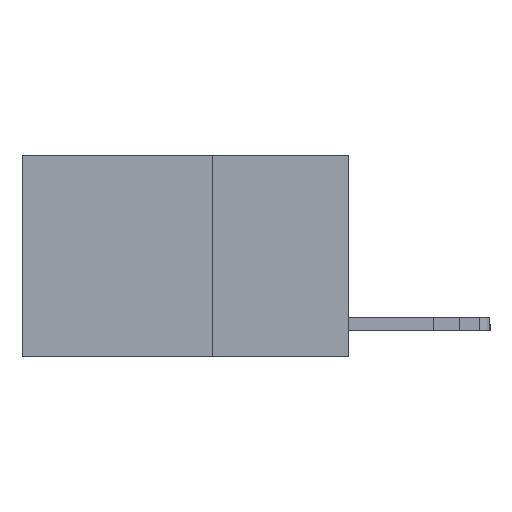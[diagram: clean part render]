
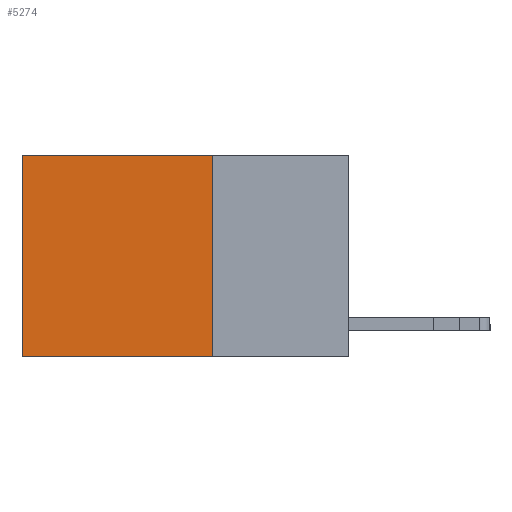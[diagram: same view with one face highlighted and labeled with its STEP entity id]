
A CAD part, left-side view. The second image highlights one B-rep face of the part: STEP entity #5274.
In plain terms, the highlighted planar face has unit normal (-1, 0, 0).
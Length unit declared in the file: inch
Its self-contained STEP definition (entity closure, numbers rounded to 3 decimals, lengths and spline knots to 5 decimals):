
#613 = VERTEX_POINT ( 'NONE', #13462 ) ;
#965 = CARTESIAN_POINT ( 'NONE',  ( 0.2625, 0.25, 0. ) ) ;
#1914 = EDGE_CURVE ( 'NONE', #18577, #613, #13755, .T. ) ;
#2426 = AXIS2_PLACEMENT_3D ( 'NONE', #17594, #7298, #4299 ) ;
#2745 = VECTOR ( 'NONE', #12208, 39.37008 ) ;
#2809 = LINE ( 'NONE', #18819, #14196 ) ;
#4299 = DIRECTION ( 'NONE',  ( 0., 0., -1. ) ) ;
#4348 = CARTESIAN_POINT ( 'NONE',  ( 0.2625, 0.25, -0.37 ) ) ;
#4615 = EDGE_CURVE ( 'NONE', #16564, #18577, #9957, .T. ) ;
#5274 = ADVANCED_FACE ( 'NONE', ( #11670 ), #14673, .F. ) ;
#5416 = DIRECTION ( 'NONE',  ( 0., 1., 0. ) ) ;
#7030 = EDGE_LOOP ( 'NONE', ( #14789, #12630, #12229, #9742 ) ) ;
#7270 = VECTOR ( 'NONE', #17537, 39.37008 ) ;
#7298 = DIRECTION ( 'NONE',  ( 1., 0., 0. ) ) ;
#7419 = EDGE_CURVE ( 'NONE', #11851, #613, #2809, .T. ) ;
#7636 = CARTESIAN_POINT ( 'NONE',  ( 0.2625, 0.6, 0. ) ) ;
#8005 = LINE ( 'NONE', #15856, #15349 ) ;
#9742 = ORIENTED_EDGE ( 'NONE', *, *, #4615, .T. ) ;
#9957 = LINE ( 'NONE', #18812, #7270 ) ;
#11670 = FACE_OUTER_BOUND ( 'NONE', #7030, .T. ) ;
#11851 = VERTEX_POINT ( 'NONE', #4348 ) ;
#12208 = DIRECTION ( 'NONE',  ( 0., 0., -1. ) ) ;
#12229 = ORIENTED_EDGE ( 'NONE', *, *, #16948, .F. ) ;
#12630 = ORIENTED_EDGE ( 'NONE', *, *, #7419, .F. ) ;
#13462 = CARTESIAN_POINT ( 'NONE',  ( 0.2625, 0.6, -0.37 ) ) ;
#13755 = LINE ( 'NONE', #7636, #2745 ) ;
#14196 = VECTOR ( 'NONE', #5416, 39.37008 ) ;
#14673 = PLANE ( 'NONE',  #2426 ) ;
#14789 = ORIENTED_EDGE ( 'NONE', *, *, #1914, .T. ) ;
#15349 = VECTOR ( 'NONE', #18781, 39.37008 ) ;
#15856 = CARTESIAN_POINT ( 'NONE',  ( 0.2625, 0.25, 0. ) ) ;
#16564 = VERTEX_POINT ( 'NONE', #965 ) ;
#16588 = CARTESIAN_POINT ( 'NONE',  ( 0.2625, 0.6, 0. ) ) ;
#16948 = EDGE_CURVE ( 'NONE', #16564, #11851, #8005, .T. ) ;
#17537 = DIRECTION ( 'NONE',  ( 0., 1., 0. ) ) ;
#17594 = CARTESIAN_POINT ( 'NONE',  ( 0.2625, 0.25, 0. ) ) ;
#18577 = VERTEX_POINT ( 'NONE', #16588 ) ;
#18781 = DIRECTION ( 'NONE',  ( 0., 0., -1. ) ) ;
#18812 = CARTESIAN_POINT ( 'NONE',  ( 0.2625, 0.25, 0. ) ) ;
#18819 = CARTESIAN_POINT ( 'NONE',  ( 0.2625, 0.25, -0.37 ) ) ;
